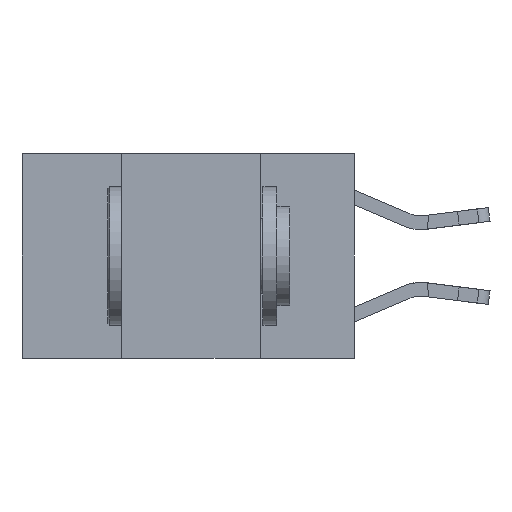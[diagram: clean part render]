
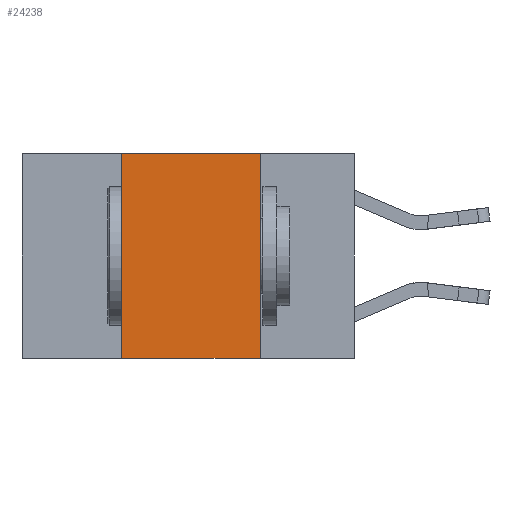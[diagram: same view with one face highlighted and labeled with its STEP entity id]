
A CAD part, left-side view. The second image highlights one B-rep face of the part: STEP entity #24238.
In plain terms, the highlighted planar face has unit normal (-1, 0, 0).
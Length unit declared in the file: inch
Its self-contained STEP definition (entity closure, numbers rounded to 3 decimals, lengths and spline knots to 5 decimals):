
#41 = VERTEX_POINT ( 'NONE', #16537 ) ;
#227 = ORIENTED_EDGE ( 'NONE', *, *, #5300, .F. ) ;
#356 = DIRECTION ( 'NONE',  ( 0., 0., -1. ) ) ;
#1356 = VERTEX_POINT ( 'NONE', #28772 ) ;
#1481 = ORIENTED_EDGE ( 'NONE', *, *, #9379, .T. ) ;
#3207 = LINE ( 'NONE', #12160, #24716 ) ;
#3900 = VERTEX_POINT ( 'NONE', #14605 ) ;
#4441 = DIRECTION ( 'NONE',  ( 0., -1., 0. ) ) ;
#5163 = LINE ( 'NONE', #5309, #22867 ) ;
#5300 = EDGE_CURVE ( 'NONE', #3900, #41, #18751, .T. ) ;
#5309 = CARTESIAN_POINT ( 'NONE',  ( 0., 0.42, 0. ) ) ;
#6799 = DIRECTION ( 'NONE',  ( 1., 0., 0. ) ) ;
#8976 = CARTESIAN_POINT ( 'NONE',  ( 0., 0.6, -0.37 ) ) ;
#9379 = EDGE_CURVE ( 'NONE', #1356, #41, #26591, .T. ) ;
#10735 = EDGE_LOOP ( 'NONE', ( #227, #19558, #25869, #1481 ) ) ;
#10970 = VECTOR ( 'NONE', #20963, 39.37008 ) ;
#11072 = FACE_OUTER_BOUND ( 'NONE', #10735, .T. ) ;
#12157 = CARTESIAN_POINT ( 'NONE',  ( 0., 0.17, 0. ) ) ;
#12160 = CARTESIAN_POINT ( 'NONE',  ( 0., 0.6, 0. ) ) ;
#14605 = CARTESIAN_POINT ( 'NONE',  ( 0., 0.17, 0. ) ) ;
#15852 = AXIS2_PLACEMENT_3D ( 'NONE', #16201, #6799, #356 ) ;
#16201 = CARTESIAN_POINT ( 'NONE',  ( 0., 0.6, 0. ) ) ;
#16537 = CARTESIAN_POINT ( 'NONE',  ( 0., 0.17, -0.37 ) ) ;
#18751 = LINE ( 'NONE', #12157, #10970 ) ;
#19558 = ORIENTED_EDGE ( 'NONE', *, *, #23556, .F. ) ;
#20963 = DIRECTION ( 'NONE',  ( 0., 0., -1. ) ) ;
#21573 = EDGE_CURVE ( 'NONE', #1356, #26798, #5163, .T. ) ;
#21591 = CARTESIAN_POINT ( 'NONE',  ( 0., 0.42, 0. ) ) ;
#22867 = VECTOR ( 'NONE', #23211, 39.37008 ) ;
#23211 = DIRECTION ( 'NONE',  ( 0., 0., 1. ) ) ;
#23556 = EDGE_CURVE ( 'NONE', #26798, #3900, #3207, .T. ) ;
#24238 = ADVANCED_FACE ( 'NONE', ( #11072 ), #27049, .F. ) ;
#24716 = VECTOR ( 'NONE', #28135, 39.37008 ) ;
#25869 = ORIENTED_EDGE ( 'NONE', *, *, #21573, .F. ) ;
#26591 = LINE ( 'NONE', #8976, #28940 ) ;
#26798 = VERTEX_POINT ( 'NONE', #21591 ) ;
#27049 = PLANE ( 'NONE',  #15852 ) ;
#28135 = DIRECTION ( 'NONE',  ( 0., -1., 0. ) ) ;
#28772 = CARTESIAN_POINT ( 'NONE',  ( 0., 0.42, -0.37 ) ) ;
#28940 = VECTOR ( 'NONE', #4441, 39.37008 ) ;
